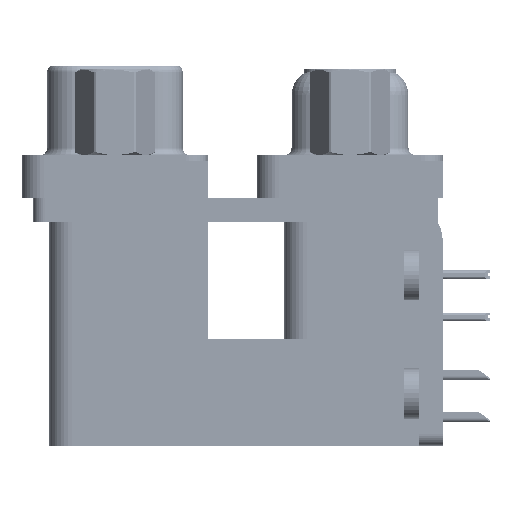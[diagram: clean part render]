
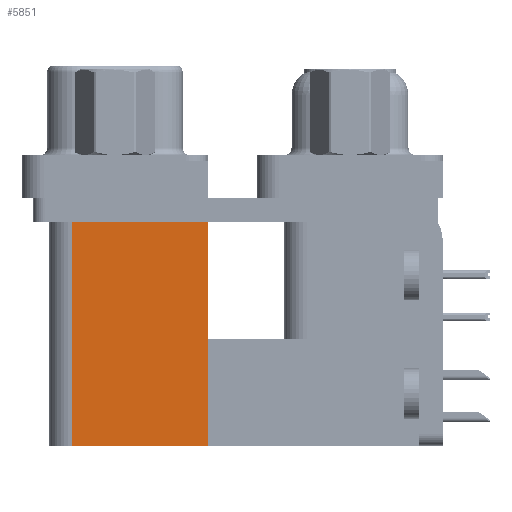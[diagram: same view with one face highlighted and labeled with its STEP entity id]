
A CAD part, left-side view. The second image highlights one B-rep face of the part: STEP entity #5851.
In plain terms, the highlighted planar face has unit normal (-1, 0, 0).
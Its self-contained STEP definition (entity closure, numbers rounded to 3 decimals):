
#4883 = ORIENTED_EDGE ( 'NONE', *, *, #51613, .T. ) ;
#5310 = VECTOR ( 'NONE', #62358, 1000. ) ;
#5851 = ADVANCED_FACE ( 'NONE', ( #30786 ), #69521, .F. ) ;
#6329 = ORIENTED_EDGE ( 'NONE', *, *, #27235, .F. ) ;
#7711 = ORIENTED_EDGE ( 'NONE', *, *, #73174, .F. ) ;
#24726 = CARTESIAN_POINT ( 'NONE',  ( 3.79, 9.6, -19.2 ) ) ;
#25968 = EDGE_LOOP ( 'NONE', ( #72279, #6329, #7711, #4883 ) ) ;
#26315 = CARTESIAN_POINT ( 'NONE',  ( 3.79, 18.8, -2.5 ) ) ;
#27235 = EDGE_CURVE ( 'NONE', #62496, #54626, #38425, .T. ) ;
#30786 = FACE_OUTER_BOUND ( 'NONE', #25968, .T. ) ;
#30940 = DIRECTION ( 'NONE',  ( 0., 1., 0. ) ) ;
#35147 = LINE ( 'NONE', #35525, #35324 ) ;
#35324 = VECTOR ( 'NONE', #30940, 1000. ) ;
#35502 = VERTEX_POINT ( 'NONE', #72638 ) ;
#35525 = CARTESIAN_POINT ( 'NONE',  ( 3.79, 9.6, -2.5 ) ) ;
#35796 = VECTOR ( 'NONE', #36374, 1000. ) ;
#36374 = DIRECTION ( 'NONE',  ( 0., 1., 0. ) ) ;
#36424 = CARTESIAN_POINT ( 'NONE',  ( 3.79, 18.8, -19.2 ) ) ;
#38425 = LINE ( 'NONE', #50964, #5310 ) ;
#42132 = LINE ( 'NONE', #53888, #57478 ) ;
#42458 = LINE ( 'NONE', #54591, #35796 ) ;
#47523 = DIRECTION ( 'NONE',  ( 1., 0., 0. ) ) ;
#47889 = DIRECTION ( 'NONE',  ( 0., 0., -1. ) ) ;
#50858 = CARTESIAN_POINT ( 'NONE',  ( 3.79, 9.6, -19.2 ) ) ;
#50964 = CARTESIAN_POINT ( 'NONE',  ( 3.79, 18.8, -19.2 ) ) ;
#51613 = EDGE_CURVE ( 'NONE', #72992, #35502, #42132, .T. ) ;
#53523 = DIRECTION ( 'NONE',  ( 0., 0., 1. ) ) ;
#53888 = CARTESIAN_POINT ( 'NONE',  ( 3.79, 9.6, -19.2 ) ) ;
#54591 = CARTESIAN_POINT ( 'NONE',  ( 3.79, 9.6, -19.2 ) ) ;
#54626 = VERTEX_POINT ( 'NONE', #26315 ) ;
#54909 = AXIS2_PLACEMENT_3D ( 'NONE', #24726, #47523, #47889 ) ;
#57478 = VECTOR ( 'NONE', #53523, 1000. ) ;
#62358 = DIRECTION ( 'NONE',  ( 0., 0., 1. ) ) ;
#62496 = VERTEX_POINT ( 'NONE', #36424 ) ;
#66494 = EDGE_CURVE ( 'NONE', #35502, #54626, #35147, .T. ) ;
#69521 = PLANE ( 'NONE',  #54909 ) ;
#72279 = ORIENTED_EDGE ( 'NONE', *, *, #66494, .T. ) ;
#72638 = CARTESIAN_POINT ( 'NONE',  ( 3.79, 9.6, -2.5 ) ) ;
#72992 = VERTEX_POINT ( 'NONE', #50858 ) ;
#73174 = EDGE_CURVE ( 'NONE', #72992, #62496, #42458, .T. ) ;
